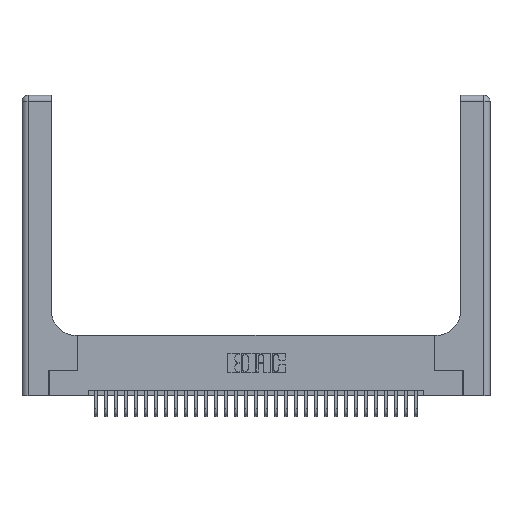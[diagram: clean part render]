
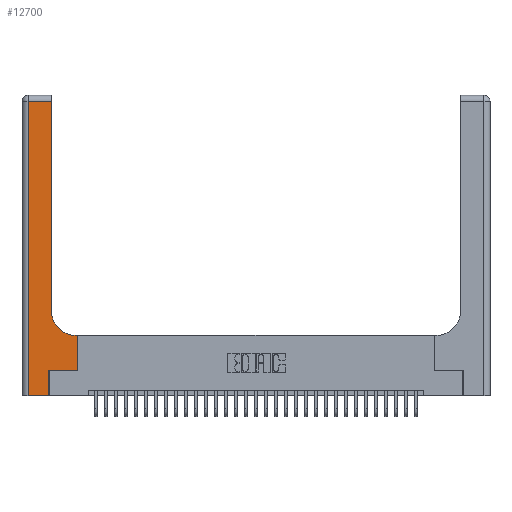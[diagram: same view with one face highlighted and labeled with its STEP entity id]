
A CAD part, top view. The second image highlights one B-rep face of the part: STEP entity #12700.
In plain terms, the highlighted planar face has unit normal (0, 0, 1).
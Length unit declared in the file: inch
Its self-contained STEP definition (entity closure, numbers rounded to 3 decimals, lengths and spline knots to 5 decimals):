
#122 = LINE ( 'NONE', #16936, #20400 ) ;
#137 = EDGE_CURVE ( 'NONE', #1509, #27714, #122, .T. ) ;
#253 = DIRECTION ( 'NONE',  ( 1., 0., 0. ) ) ;
#1274 = ORIENTED_EDGE ( 'NONE', *, *, #32610, .T. ) ;
#1448 = CARTESIAN_POINT ( 'NONE',  ( 0.5415, 0.6, 0.37 ) ) ;
#1509 = VERTEX_POINT ( 'NONE', #28099 ) ;
#1626 = PLANE ( 'NONE',  #15412 ) ;
#1738 = DIRECTION ( 'NONE',  ( 0., 0., -1. ) ) ;
#2531 = LINE ( 'NONE', #16209, #14978 ) ;
#3297 = CARTESIAN_POINT ( 'NONE',  ( 0.5585, 0.25, 0.37 ) ) ;
#3576 = ORIENTED_EDGE ( 'NONE', *, *, #31433, .T. ) ;
#3610 = DIRECTION ( 'NONE',  ( 0., 1., 0. ) ) ;
#3730 = CARTESIAN_POINT ( 'NONE',  ( 0.269, 0., 0.37 ) ) ;
#3794 = DIRECTION ( 'NONE',  ( 1., 0., 0. ) ) ;
#4277 = FACE_OUTER_BOUND ( 'NONE', #5779, .T. ) ;
#4510 = EDGE_CURVE ( 'NONE', #27714, #23640, #20801, .T. ) ;
#5103 = CIRCLE ( 'NONE', #29520, 0.25 ) ;
#5779 = EDGE_LOOP ( 'NONE', ( #3576, #9767, #31573, #20786, #17284, #8887, #10513, #17043, #1274 ) ) ;
#6647 = DIRECTION ( 'NONE',  ( -1., 0., 0. ) ) ;
#6734 = VECTOR ( 'NONE', #30194, 39.37008 ) ;
#6754 = EDGE_CURVE ( 'NONE', #31143, #1509, #7574, .T. ) ;
#7574 = LINE ( 'NONE', #11948, #6734 ) ;
#7753 = DIRECTION ( 'NONE',  ( 0., 0., -1. ) ) ;
#8887 = ORIENTED_EDGE ( 'NONE', *, *, #21232, .T. ) ;
#9273 = CARTESIAN_POINT ( 'NONE',  ( 0.2915, 0.85, 0.37 ) ) ;
#9513 = VERTEX_POINT ( 'NONE', #32371 ) ;
#9767 = ORIENTED_EDGE ( 'NONE', *, *, #27803, .T. ) ;
#10513 = ORIENTED_EDGE ( 'NONE', *, *, #17042, .T. ) ;
#10800 = VERTEX_POINT ( 'NONE', #33088 ) ;
#11948 = CARTESIAN_POINT ( 'NONE',  ( 0.06, 3., 0.37 ) ) ;
#12350 = CARTESIAN_POINT ( 'NONE',  ( 0., 3., 0.37 ) ) ;
#12700 = ADVANCED_FACE ( 'NONE', ( #4277 ), #1626, .F. ) ;
#13115 = EDGE_CURVE ( 'NONE', #10800, #30891, #19104, .T. ) ;
#13476 = VECTOR ( 'NONE', #3610, 39.37008 ) ;
#13930 = VECTOR ( 'NONE', #27875, 39.37008 ) ;
#13979 = DIRECTION ( 'NONE',  ( 0., 1., 0. ) ) ;
#14053 = CARTESIAN_POINT ( 'NONE',  ( 0.2915, 3., 0.37 ) ) ;
#14978 = VECTOR ( 'NONE', #253, 39.37008 ) ;
#15412 = AXIS2_PLACEMENT_3D ( 'NONE', #12350, #1738, #20230 ) ;
#15859 = VERTEX_POINT ( 'NONE', #9273 ) ;
#16209 = CARTESIAN_POINT ( 'NONE',  ( 0.269, 0.25, 0.37 ) ) ;
#16936 = CARTESIAN_POINT ( 'NONE',  ( 0., 0., 0.37 ) ) ;
#17042 = EDGE_CURVE ( 'NONE', #9513, #10800, #19299, .T. ) ;
#17043 = ORIENTED_EDGE ( 'NONE', *, *, #13115, .T. ) ;
#17284 = ORIENTED_EDGE ( 'NONE', *, *, #4510, .T. ) ;
#19104 = LINE ( 'NONE', #19757, #26874 ) ;
#19299 = LINE ( 'NONE', #3297, #32293 ) ;
#19542 = CARTESIAN_POINT ( 'NONE',  ( 0.269, 0., 0.37 ) ) ;
#19757 = CARTESIAN_POINT ( 'NONE',  ( 0.2915, 0.6, 0.37 ) ) ;
#20230 = DIRECTION ( 'NONE',  ( -1., 0., 0. ) ) ;
#20400 = VECTOR ( 'NONE', #3794, 39.37008 ) ;
#20786 = ORIENTED_EDGE ( 'NONE', *, *, #137, .T. ) ;
#20801 = LINE ( 'NONE', #3730, #33766 ) ;
#21046 = CARTESIAN_POINT ( 'NONE',  ( 0.269, 0.25, 0.37 ) ) ;
#21232 = EDGE_CURVE ( 'NONE', #23640, #9513, #2531, .T. ) ;
#21295 = CARTESIAN_POINT ( 'NONE',  ( 0.2915, 2.94, 0.37 ) ) ;
#23473 = CARTESIAN_POINT ( 'NONE',  ( 0.5415, 0.85, 0.37 ) ) ;
#23640 = VERTEX_POINT ( 'NONE', #21046 ) ;
#25250 = CARTESIAN_POINT ( 'NONE',  ( 0., 2.94, 0.37 ) ) ;
#26070 = CARTESIAN_POINT ( 'NONE',  ( 0.06, 2.94, 0.37 ) ) ;
#26078 = DIRECTION ( 'NONE',  ( 1., 0., 0. ) ) ;
#26874 = VECTOR ( 'NONE', #6647, 39.37008 ) ;
#26922 = VERTEX_POINT ( 'NONE', #21295 ) ;
#27392 = LINE ( 'NONE', #14053, #13476 ) ;
#27436 = DIRECTION ( 'NONE',  ( 0., 1., 0. ) ) ;
#27714 = VERTEX_POINT ( 'NONE', #19542 ) ;
#27803 = EDGE_CURVE ( 'NONE', #26922, #31143, #27859, .T. ) ;
#27859 = LINE ( 'NONE', #25250, #13930 ) ;
#27875 = DIRECTION ( 'NONE',  ( -1., 0., 0. ) ) ;
#28099 = CARTESIAN_POINT ( 'NONE',  ( 0.06, 0., 0.37 ) ) ;
#29520 = AXIS2_PLACEMENT_3D ( 'NONE', #23473, #7753, #26078 ) ;
#30194 = DIRECTION ( 'NONE',  ( 0., -1., 0. ) ) ;
#30891 = VERTEX_POINT ( 'NONE', #1448 ) ;
#31143 = VERTEX_POINT ( 'NONE', #26070 ) ;
#31433 = EDGE_CURVE ( 'NONE', #15859, #26922, #27392, .T. ) ;
#31573 = ORIENTED_EDGE ( 'NONE', *, *, #6754, .T. ) ;
#32293 = VECTOR ( 'NONE', #13979, 39.37008 ) ;
#32371 = CARTESIAN_POINT ( 'NONE',  ( 0.5585, 0.25, 0.37 ) ) ;
#32610 = EDGE_CURVE ( 'NONE', #30891, #15859, #5103, .T. ) ;
#33088 = CARTESIAN_POINT ( 'NONE',  ( 0.5585, 0.6, 0.37 ) ) ;
#33766 = VECTOR ( 'NONE', #27436, 39.37008 ) ;
